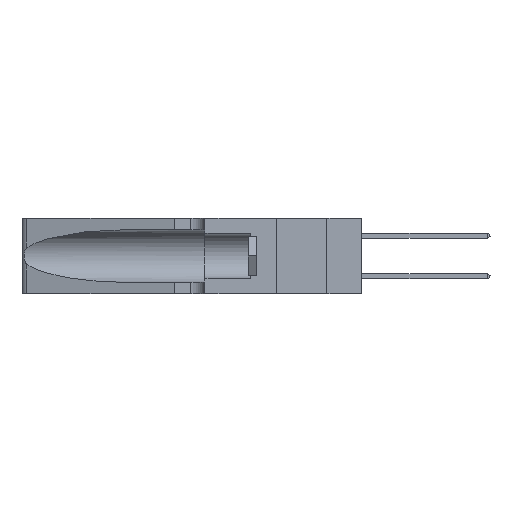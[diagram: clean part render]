
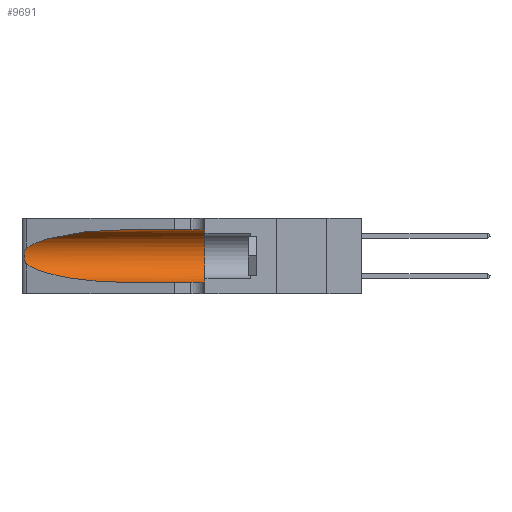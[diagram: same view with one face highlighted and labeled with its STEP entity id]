
A CAD part, left-side view. The second image highlights one B-rep face of the part: STEP entity #9691.
In plain terms, the highlighted cylindrical face has radius 3.308 mm (diameter 6.617 mm), a partial arc.
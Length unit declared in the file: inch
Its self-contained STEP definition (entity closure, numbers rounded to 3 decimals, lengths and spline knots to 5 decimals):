
#359 = CARTESIAN_POINT ( 'NONE',  ( 0.26075, 1.23896, 0.19203 ) ) ;
#1449 = LINE ( 'NONE', #21479, #18199 ) ;
#1796 = VERTEX_POINT ( 'NONE', #37960 ) ;
#2157 = EDGE_CURVE ( 'NONE', #35271, #5875, #1449, .T. ) ;
#2541 = CARTESIAN_POINT ( 'NONE',  ( 0.2373, 1.15595, 0.08982 ) ) ;
#2673 = DIRECTION ( 'NONE',  ( 0., -1., 0. ) ) ;
#2932 = VERTEX_POINT ( 'NONE', #9417 ) ;
#3557 = CARTESIAN_POINT ( 'NONE',  ( 0.26017, 1.23833, 0.17102 ) ) ;
#3937 = B_SPLINE_CURVE_WITH_KNOTS ( 'NONE', 3,
 ( #9794, #28497, #34728, #16085, #37830, #19246, #359, #22354, #3557, #25478, #6768, #28631, #9935, #31751 ),
 .UNSPECIFIED., .F., .F.,
 ( 4, 2, 2, 2, 2, 2, 4 ),
 ( 0., 0.00027, 0.00053, 0.00107, 0.0016, 0.00187, 0.00214 ),
 .UNSPECIFIED. ) ;
#4555 = ORIENTED_EDGE ( 'NONE', *, *, #35916, .T. ) ;
#5875 = VERTEX_POINT ( 'NONE', #27814 ) ;
#5894 = DIRECTION ( 'NONE',  ( 0., 0., -1. ) ) ;
#6536 = EDGE_CURVE ( 'NONE', #1796, #35271, #10640, .T. ) ;
#6562 = ORIENTED_EDGE ( 'NONE', *, *, #9257, .T. ) ;
#6768 = CARTESIAN_POINT ( 'NONE',  ( 0.25789, 1.23486, 0.15765 ) ) ;
#7975 = FACE_OUTER_BOUND ( 'NONE', #27505, .T. ) ;
#8407 = DIRECTION ( 'NONE',  ( 0., -1., 0. ) ) ;
#8493 = EDGE_CURVE ( 'NONE', #2932, #5875, #34476, .T. ) ;
#9257 = EDGE_CURVE ( 'NONE', #19024, #1796, #3937, .T. ) ;
#9417 = CARTESIAN_POINT ( 'NONE',  ( 0.1305, 0.35, 0.31525 ) ) ;
#9446 = AXIS2_PLACEMENT_3D ( 'NONE', #28268, #9559, #31389 ) ;
#9559 = DIRECTION ( 'NONE',  ( 0., 1., 0. ) ) ;
#9691 = ADVANCED_FACE ( 'NONE', ( #7975 ), #21661, .F. ) ;
#9794 = CARTESIAN_POINT ( 'NONE',  ( 0.25487, 1.22718, 0.22369 ) ) ;
#9935 = CARTESIAN_POINT ( 'NONE',  ( 0.25555, 1.22993, 0.14849 ) ) ;
#10640 =( BOUNDED_CURVE ( )  B_SPLINE_CURVE ( 3, ( #27622, #2541, #30764, #12068 ),
 .UNSPECIFIED., .F., .F. ) 
 B_SPLINE_CURVE_WITH_KNOTS ( ( 4, 4 ),
 ( 3.44316, 4.71239 ),
 .UNSPECIFIED. ) 
 CURVE ( )  GEOMETRIC_REPRESENTATION_ITEM ( )  RATIONAL_B_SPLINE_CURVE ( ( 1., 0.87, 0.87, 1. ) ) 
 REPRESENTATION_ITEM ( '' )  );
#11346 = CARTESIAN_POINT ( 'NONE',  ( 0.1305, 0.72297, 0.31525 ) ) ;
#12068 = CARTESIAN_POINT ( 'NONE',  ( 0.1305, 0.72297, 0.05475 ) ) ;
#12564 = EDGE_CURVE ( 'NONE', #34788, #2932, #38681, .T. ) ;
#14508 = CARTESIAN_POINT ( 'NONE',  ( 0.2373, 1.15595, 0.28018 ) ) ;
#14555 =( BOUNDED_CURVE ( )  B_SPLINE_CURVE ( 3, ( #11346, #20651, #14508, #36284 ),
 .UNSPECIFIED., .F., .F. ) 
 B_SPLINE_CURVE_WITH_KNOTS ( ( 4, 4 ),
 ( 1.5708, 2.84003 ),
 .UNSPECIFIED. ) 
 CURVE ( )  GEOMETRIC_REPRESENTATION_ITEM ( )  RATIONAL_B_SPLINE_CURVE ( ( 1., 0.87, 0.87, 1. ) ) 
 REPRESENTATION_ITEM ( '' )  );
#14850 = VECTOR ( 'NONE', #8407, 39.37008 ) ;
#16085 = CARTESIAN_POINT ( 'NONE',  ( 0.25787, 1.23484, 0.2124 ) ) ;
#16344 = CARTESIAN_POINT ( 'NONE',  ( 0.25487, 1.22718, 0.22369 ) ) ;
#17830 = ORIENTED_EDGE ( 'NONE', *, *, #12564, .F. ) ;
#18199 = VECTOR ( 'NONE', #2673, 39.37008 ) ;
#19024 = VERTEX_POINT ( 'NONE', #16344 ) ;
#19246 = CARTESIAN_POINT ( 'NONE',  ( 0.26018, 1.23835, 0.19895 ) ) ;
#20651 = CARTESIAN_POINT ( 'NONE',  ( 0.18966, 0.96281, 0.31525 ) ) ;
#21479 = CARTESIAN_POINT ( 'NONE',  ( 0.1305, 1.61858, 0.05475 ) ) ;
#21661 = CYLINDRICAL_SURFACE ( 'NONE', #25927, 0.13025 ) ;
#22354 = CARTESIAN_POINT ( 'NONE',  ( 0.26075, 1.23896, 0.178 ) ) ;
#23176 = ORIENTED_EDGE ( 'NONE', *, *, #6536, .T. ) ;
#23980 = CARTESIAN_POINT ( 'NONE',  ( 0.1305, 1.61858, 0.31525 ) ) ;
#25126 = ORIENTED_EDGE ( 'NONE', *, *, #8493, .F. ) ;
#25478 = CARTESIAN_POINT ( 'NONE',  ( 0.25856, 1.23593, 0.16098 ) ) ;
#25927 = AXIS2_PLACEMENT_3D ( 'NONE', #27762, #34015, #5894 ) ;
#27505 = EDGE_LOOP ( 'NONE', ( #4555, #6562, #23176, #39674, #25126, #17830 ) ) ;
#27622 = CARTESIAN_POINT ( 'NONE',  ( 0.25487, 1.22718, 0.14631 ) ) ;
#27762 = CARTESIAN_POINT ( 'NONE',  ( 0.1305, 1.61858, 0.185 ) ) ;
#27814 = CARTESIAN_POINT ( 'NONE',  ( 0.1305, 0.35, 0.05475 ) ) ;
#28268 = CARTESIAN_POINT ( 'NONE',  ( 0.1305, 0.35, 0.185 ) ) ;
#28497 = CARTESIAN_POINT ( 'NONE',  ( 0.25555, 1.22994, 0.2215 ) ) ;
#28631 = CARTESIAN_POINT ( 'NONE',  ( 0.25639, 1.23186, 0.15144 ) ) ;
#30764 = CARTESIAN_POINT ( 'NONE',  ( 0.18966, 0.96281, 0.05475 ) ) ;
#31389 = DIRECTION ( 'NONE',  ( 0., 0., 1. ) ) ;
#31751 = CARTESIAN_POINT ( 'NONE',  ( 0.25487, 1.22718, 0.14631 ) ) ;
#34015 = DIRECTION ( 'NONE',  ( 0., -1., 0. ) ) ;
#34476 = CIRCLE ( 'NONE', #9446, 0.13025 ) ;
#34728 = CARTESIAN_POINT ( 'NONE',  ( 0.25639, 1.23184, 0.21858 ) ) ;
#34788 = VERTEX_POINT ( 'NONE', #40134 ) ;
#35271 = VERTEX_POINT ( 'NONE', #36198 ) ;
#35916 = EDGE_CURVE ( 'NONE', #34788, #19024, #14555, .T. ) ;
#36198 = CARTESIAN_POINT ( 'NONE',  ( 0.1305, 0.72297, 0.05475 ) ) ;
#36284 = CARTESIAN_POINT ( 'NONE',  ( 0.25487, 1.22718, 0.22369 ) ) ;
#37830 = CARTESIAN_POINT ( 'NONE',  ( 0.25854, 1.2359, 0.20912 ) ) ;
#37960 = CARTESIAN_POINT ( 'NONE',  ( 0.25487, 1.22718, 0.14631 ) ) ;
#38681 = LINE ( 'NONE', #23980, #14850 ) ;
#39674 = ORIENTED_EDGE ( 'NONE', *, *, #2157, .T. ) ;
#40134 = CARTESIAN_POINT ( 'NONE',  ( 0.1305, 0.72297, 0.31525 ) ) ;
